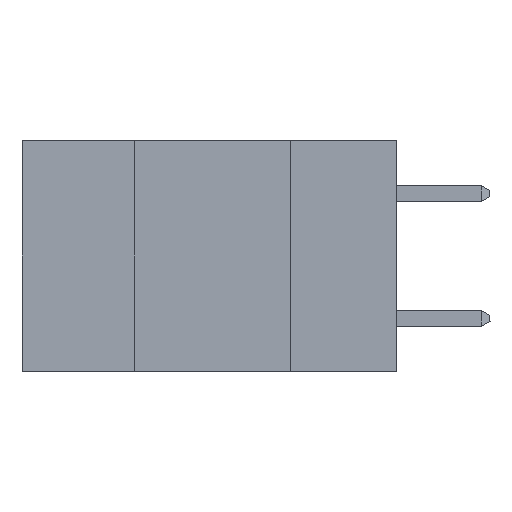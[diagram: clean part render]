
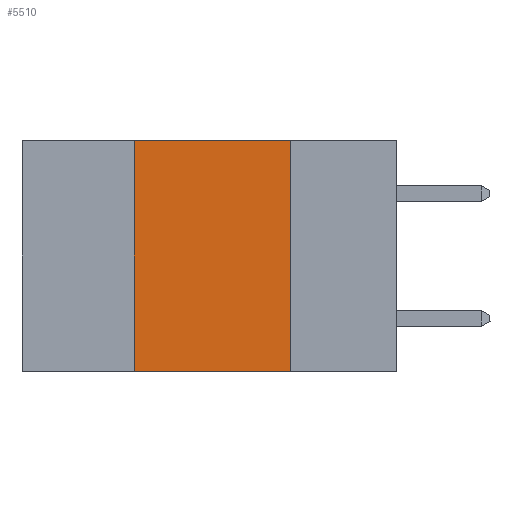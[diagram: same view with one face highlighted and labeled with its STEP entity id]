
A CAD part, left-side view. The second image highlights one B-rep face of the part: STEP entity #5510.
In plain terms, the highlighted planar face has unit normal (-1, 0, 0).
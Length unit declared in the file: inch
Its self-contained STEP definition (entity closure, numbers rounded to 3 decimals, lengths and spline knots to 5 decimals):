
#537 = DIRECTION ( 'NONE',  ( 1., 0., 0. ) ) ;
#827 = ORIENTED_EDGE ( 'NONE', *, *, #7561, .F. ) ;
#916 = LINE ( 'NONE', #1474, #1633 ) ;
#1159 = EDGE_LOOP ( 'NONE', ( #827, #4515, #6157, #11679 ) ) ;
#1474 = CARTESIAN_POINT ( 'NONE',  ( 0., 0.6, 0. ) ) ;
#1633 = VECTOR ( 'NONE', #10651, 39.37008 ) ;
#2246 = CARTESIAN_POINT ( 'NONE',  ( 0., 0.42, 0. ) ) ;
#2299 = AXIS2_PLACEMENT_3D ( 'NONE', #4707, #537, #9797 ) ;
#2885 = FACE_OUTER_BOUND ( 'NONE', #1159, .T. ) ;
#3101 = VERTEX_POINT ( 'NONE', #5375 ) ;
#3297 = DIRECTION ( 'NONE',  ( 0., -1., 0. ) ) ;
#4244 = CARTESIAN_POINT ( 'NONE',  ( 0., 0.17, -0.37 ) ) ;
#4459 = EDGE_CURVE ( 'NONE', #3101, #5240, #7356, .T. ) ;
#4461 = EDGE_CURVE ( 'NONE', #5240, #10263, #916, .T. ) ;
#4515 = ORIENTED_EDGE ( 'NONE', *, *, #4461, .F. ) ;
#4707 = CARTESIAN_POINT ( 'NONE',  ( 0., 0.6, 0. ) ) ;
#5129 = LINE ( 'NONE', #6845, #6700 ) ;
#5240 = VERTEX_POINT ( 'NONE', #2246 ) ;
#5375 = CARTESIAN_POINT ( 'NONE',  ( 0., 0.42, -0.37 ) ) ;
#5392 = LINE ( 'NONE', #6009, #11929 ) ;
#5510 = ADVANCED_FACE ( 'NONE', ( #2885 ), #9119, .F. ) ;
#6009 = CARTESIAN_POINT ( 'NONE',  ( 0., 0.17, 0. ) ) ;
#6046 = DIRECTION ( 'NONE',  ( 0., 0., -1. ) ) ;
#6157 = ORIENTED_EDGE ( 'NONE', *, *, #4459, .F. ) ;
#6700 = VECTOR ( 'NONE', #3297, 39.37008 ) ;
#6704 = CARTESIAN_POINT ( 'NONE',  ( 0., 0.17, 0. ) ) ;
#6845 = CARTESIAN_POINT ( 'NONE',  ( 0., 0.6, -0.37 ) ) ;
#7356 = LINE ( 'NONE', #8692, #8069 ) ;
#7419 = EDGE_CURVE ( 'NONE', #3101, #7957, #5129, .T. ) ;
#7561 = EDGE_CURVE ( 'NONE', #10263, #7957, #5392, .T. ) ;
#7771 = DIRECTION ( 'NONE',  ( 0., 0., 1. ) ) ;
#7957 = VERTEX_POINT ( 'NONE', #4244 ) ;
#8069 = VECTOR ( 'NONE', #7771, 39.37008 ) ;
#8692 = CARTESIAN_POINT ( 'NONE',  ( 0., 0.42, 0. ) ) ;
#9119 = PLANE ( 'NONE',  #2299 ) ;
#9797 = DIRECTION ( 'NONE',  ( 0., 0., -1. ) ) ;
#10263 = VERTEX_POINT ( 'NONE', #6704 ) ;
#10651 = DIRECTION ( 'NONE',  ( 0., -1., 0. ) ) ;
#11679 = ORIENTED_EDGE ( 'NONE', *, *, #7419, .T. ) ;
#11929 = VECTOR ( 'NONE', #6046, 39.37008 ) ;
